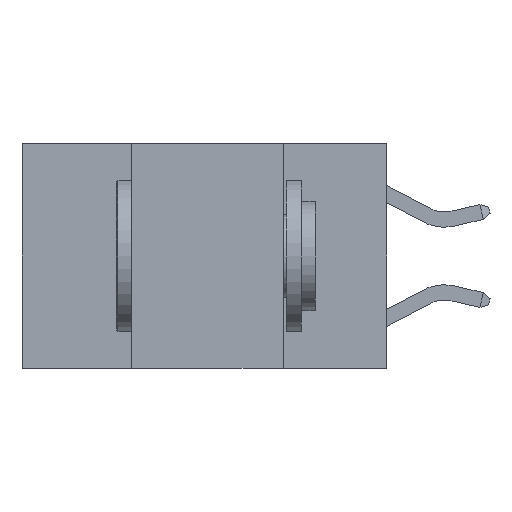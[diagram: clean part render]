
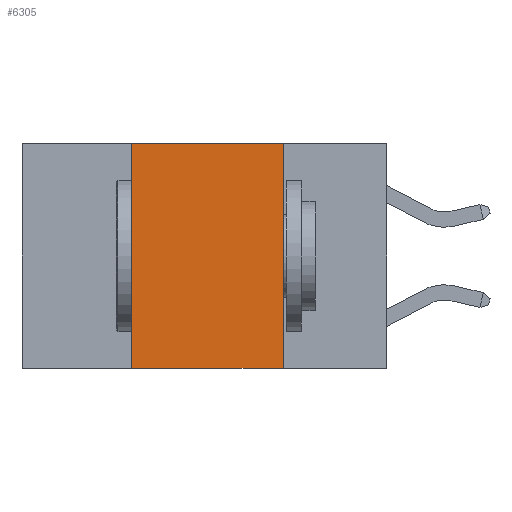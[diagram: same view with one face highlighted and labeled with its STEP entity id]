
A CAD part, left-side view. The second image highlights one B-rep face of the part: STEP entity #6305.
In plain terms, the highlighted planar face has unit normal (-1, 0, 0).
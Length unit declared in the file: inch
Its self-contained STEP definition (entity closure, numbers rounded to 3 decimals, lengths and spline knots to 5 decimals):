
#353 = VECTOR ( 'NONE', #5397, 39.37008 ) ;
#443 = ORIENTED_EDGE ( 'NONE', *, *, #10353, .T. ) ;
#537 = CARTESIAN_POINT ( 'NONE',  ( 0., 0.42, 0. ) ) ;
#603 = FACE_OUTER_BOUND ( 'NONE', #10347, .T. ) ;
#887 = CARTESIAN_POINT ( 'NONE',  ( 0., 0.42, -0.37 ) ) ;
#1602 = DIRECTION ( 'NONE',  ( 0., 0., 1. ) ) ;
#2466 = CARTESIAN_POINT ( 'NONE',  ( 0., 0.6, -0.37 ) ) ;
#2787 = CARTESIAN_POINT ( 'NONE',  ( 0., 0.6, 0. ) ) ;
#3212 = CARTESIAN_POINT ( 'NONE',  ( 0., 0.17, 0. ) ) ;
#3625 = CARTESIAN_POINT ( 'NONE',  ( 0., 0.42, 0. ) ) ;
#3880 = VECTOR ( 'NONE', #1602, 39.37008 ) ;
#4601 = DIRECTION ( 'NONE',  ( 1., 0., 0. ) ) ;
#4746 = VERTEX_POINT ( 'NONE', #3212 ) ;
#5094 = EDGE_CURVE ( 'NONE', #10624, #4746, #11624, .T. ) ;
#5288 = LINE ( 'NONE', #11941, #8359 ) ;
#5397 = DIRECTION ( 'NONE',  ( 0., -1., 0. ) ) ;
#5448 = LINE ( 'NONE', #537, #3880 ) ;
#6305 = ADVANCED_FACE ( 'NONE', ( #603 ), #6396, .F. ) ;
#6338 = CARTESIAN_POINT ( 'NONE',  ( 0., 0.6, 0. ) ) ;
#6350 = EDGE_CURVE ( 'NONE', #7354, #10624, #5448, .T. ) ;
#6362 = ORIENTED_EDGE ( 'NONE', *, *, #5094, .F. ) ;
#6396 = PLANE ( 'NONE',  #8809 ) ;
#6836 = EDGE_CURVE ( 'NONE', #4746, #8737, #5288, .T. ) ;
#6931 = VECTOR ( 'NONE', #7610, 39.37008 ) ;
#7354 = VERTEX_POINT ( 'NONE', #887 ) ;
#7439 = DIRECTION ( 'NONE',  ( 0., 0., -1. ) ) ;
#7576 = LINE ( 'NONE', #2466, #353 ) ;
#7610 = DIRECTION ( 'NONE',  ( 0., -1., 0. ) ) ;
#8119 = DIRECTION ( 'NONE',  ( 0., 0., -1. ) ) ;
#8359 = VECTOR ( 'NONE', #8119, 39.37008 ) ;
#8375 = CARTESIAN_POINT ( 'NONE',  ( 0., 0.17, -0.37 ) ) ;
#8737 = VERTEX_POINT ( 'NONE', #8375 ) ;
#8809 = AXIS2_PLACEMENT_3D ( 'NONE', #6338, #4601, #7439 ) ;
#10347 = EDGE_LOOP ( 'NONE', ( #11658, #6362, #12250, #443 ) ) ;
#10353 = EDGE_CURVE ( 'NONE', #7354, #8737, #7576, .T. ) ;
#10624 = VERTEX_POINT ( 'NONE', #3625 ) ;
#11624 = LINE ( 'NONE', #2787, #6931 ) ;
#11658 = ORIENTED_EDGE ( 'NONE', *, *, #6836, .F. ) ;
#11941 = CARTESIAN_POINT ( 'NONE',  ( 0., 0.17, 0. ) ) ;
#12250 = ORIENTED_EDGE ( 'NONE', *, *, #6350, .F. ) ;
